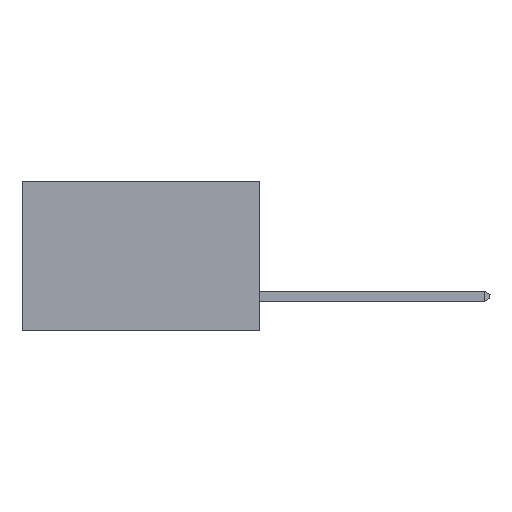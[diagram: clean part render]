
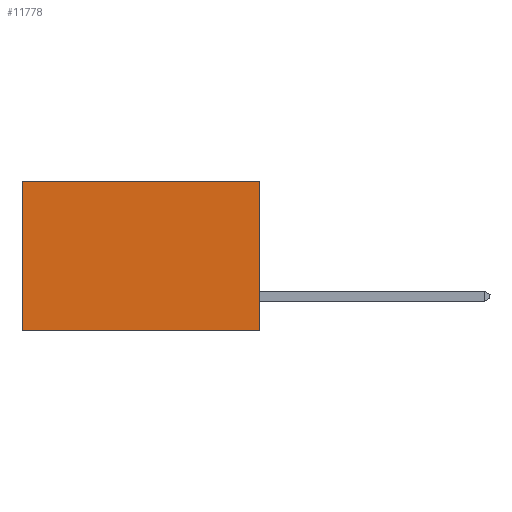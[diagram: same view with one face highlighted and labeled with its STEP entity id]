
A CAD part, left-side view. The second image highlights one B-rep face of the part: STEP entity #11778.
In plain terms, the highlighted planar face has unit normal (-1, 0, 0).
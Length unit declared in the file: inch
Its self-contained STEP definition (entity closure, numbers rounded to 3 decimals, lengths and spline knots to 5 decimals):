
#822 = ORIENTED_EDGE ( 'NONE', *, *, #3763, .F. ) ;
#1425 = CARTESIAN_POINT ( 'NONE',  ( 0.277, 0., 0. ) ) ;
#2360 = PLANE ( 'NONE',  #8434 ) ;
#2940 = LINE ( 'NONE', #8568, #10854 ) ;
#2975 = VERTEX_POINT ( 'NONE', #12843 ) ;
#3314 = CARTESIAN_POINT ( 'NONE',  ( 0.277, 0., -0.37 ) ) ;
#3319 = DIRECTION ( 'NONE',  ( 0., 0., -1. ) ) ;
#3365 = ORIENTED_EDGE ( 'NONE', *, *, #3638, .F. ) ;
#3638 = EDGE_CURVE ( 'NONE', #11303, #9730, #11048, .T. ) ;
#3700 = ORIENTED_EDGE ( 'NONE', *, *, #7571, .T. ) ;
#3763 = EDGE_CURVE ( 'NONE', #2975, #11303, #9000, .T. ) ;
#4256 = VERTEX_POINT ( 'NONE', #9286 ) ;
#5208 = CARTESIAN_POINT ( 'NONE',  ( 0.277, 0., -0.37 ) ) ;
#5516 = DIRECTION ( 'NONE',  ( 1., 0., 0. ) ) ;
#7368 = EDGE_LOOP ( 'NONE', ( #11214, #3365, #822, #3700 ) ) ;
#7403 = FACE_OUTER_BOUND ( 'NONE', #7368, .T. ) ;
#7571 = EDGE_CURVE ( 'NONE', #2975, #4256, #11415, .T. ) ;
#7911 = EDGE_CURVE ( 'NONE', #4256, #9730, #2940, .T. ) ;
#8434 = AXIS2_PLACEMENT_3D ( 'NONE', #11545, #5516, #12419 ) ;
#8487 = VECTOR ( 'NONE', #11909, 39.37008 ) ;
#8568 = CARTESIAN_POINT ( 'NONE',  ( 0.277, 0.59, -0.37 ) ) ;
#9000 = LINE ( 'NONE', #3314, #10898 ) ;
#9286 = CARTESIAN_POINT ( 'NONE',  ( 0.277, 0.59, 0. ) ) ;
#9640 = DIRECTION ( 'NONE',  ( 0., 0., -1. ) ) ;
#9730 = VERTEX_POINT ( 'NONE', #11072 ) ;
#9893 = DIRECTION ( 'NONE',  ( 0., 1., 0. ) ) ;
#10854 = VECTOR ( 'NONE', #9640, 39.37008 ) ;
#10898 = VECTOR ( 'NONE', #3319, 39.37008 ) ;
#11048 = LINE ( 'NONE', #12616, #8487 ) ;
#11072 = CARTESIAN_POINT ( 'NONE',  ( 0.277, 0.59, -0.37 ) ) ;
#11145 = VECTOR ( 'NONE', #9893, 39.37008 ) ;
#11214 = ORIENTED_EDGE ( 'NONE', *, *, #7911, .T. ) ;
#11303 = VERTEX_POINT ( 'NONE', #5208 ) ;
#11415 = LINE ( 'NONE', #1425, #11145 ) ;
#11545 = CARTESIAN_POINT ( 'NONE',  ( 0.277, 0., -0.37 ) ) ;
#11778 = ADVANCED_FACE ( 'NONE', ( #7403 ), #2360, .F. ) ;
#11909 = DIRECTION ( 'NONE',  ( 0., 1., 0. ) ) ;
#12419 = DIRECTION ( 'NONE',  ( 0., 0., -1. ) ) ;
#12616 = CARTESIAN_POINT ( 'NONE',  ( 0.277, 0., -0.37 ) ) ;
#12843 = CARTESIAN_POINT ( 'NONE',  ( 0.277, 0., 0. ) ) ;
